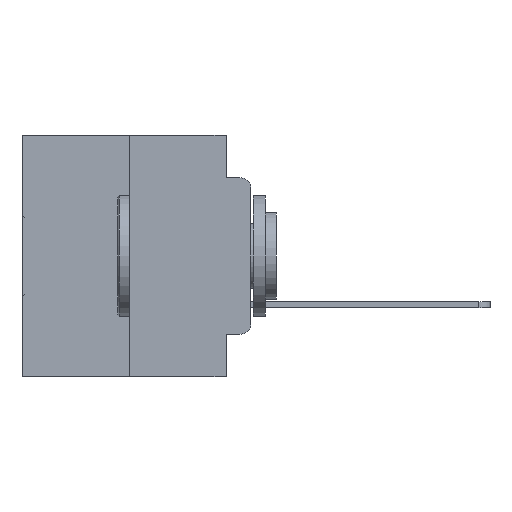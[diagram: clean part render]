
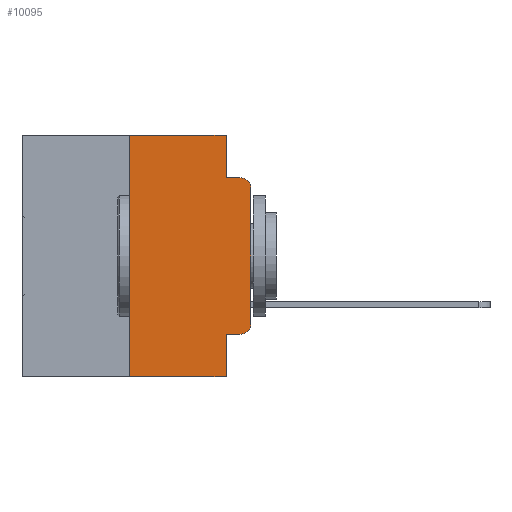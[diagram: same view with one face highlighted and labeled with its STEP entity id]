
A CAD part, left-side view. The second image highlights one B-rep face of the part: STEP entity #10095.
In plain terms, the highlighted planar face has unit normal (-1, 0, 0).
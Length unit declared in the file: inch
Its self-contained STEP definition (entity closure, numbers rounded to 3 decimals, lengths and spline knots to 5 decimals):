
#106 = DIRECTION ( 'NONE',  ( 0., 0., -1. ) ) ;
#397 = CARTESIAN_POINT ( 'NONE',  ( 0., 0., -0.3915 ) ) ;
#846 = CARTESIAN_POINT ( 'NONE',  ( 0., 0.25, 0. ) ) ;
#1183 = CARTESIAN_POINT ( 'NONE',  ( 0., 0.473, 0. ) ) ;
#2488 = CIRCLE ( 'NONE', #30219, 0.02 ) ;
#3315 = CARTESIAN_POINT ( 'NONE',  ( 0., 0.051, 0. ) ) ;
#3366 = LINE ( 'NONE', #1183, #28882 ) ;
#3495 = PLANE ( 'NONE',  #21438 ) ;
#3623 = DIRECTION ( 'NONE',  ( 0., 0., 1. ) ) ;
#3727 = LINE ( 'NONE', #16017, #16813 ) ;
#4218 = VECTOR ( 'NONE', #6435, 39.37008 ) ;
#4271 = VERTEX_POINT ( 'NONE', #10151 ) ;
#4418 = VERTEX_POINT ( 'NONE', #397 ) ;
#6343 = CARTESIAN_POINT ( 'NONE',  ( 0., 0.051, -0.0885 ) ) ;
#6427 = EDGE_CURVE ( 'NONE', #24190, #14633, #23889, .T. ) ;
#6435 = DIRECTION ( 'NONE',  ( 0., -1., 0. ) ) ;
#6467 = EDGE_CURVE ( 'NONE', #20273, #17217, #3366, .T. ) ;
#8149 = CARTESIAN_POINT ( 'NONE',  ( 0., 0.051, -0.5 ) ) ;
#8828 = DIRECTION ( 'NONE',  ( 0., 0., -1. ) ) ;
#9585 = DIRECTION ( 'NONE',  ( -1., 0., 0. ) ) ;
#10095 = ADVANCED_FACE ( 'NONE', ( #21127 ), #3495, .F. ) ;
#10151 = CARTESIAN_POINT ( 'NONE',  ( 0., 0., -0.1085 ) ) ;
#11311 = EDGE_LOOP ( 'NONE', ( #19283, #19315, #19781, #19879, #20159, #20254, #20561, #20663, #20999, #21186 ) ) ;
#11604 = VERTEX_POINT ( 'NONE', #26144 ) ;
#12731 = EDGE_CURVE ( 'NONE', #24190, #28984, #3727, .T. ) ;
#13324 = CARTESIAN_POINT ( 'NONE',  ( 0., 0.25, 0. ) ) ;
#14471 = EDGE_CURVE ( 'NONE', #11604, #20273, #20248, .T. ) ;
#14633 = VERTEX_POINT ( 'NONE', #24631 ) ;
#15648 = VECTOR ( 'NONE', #20537, 39.37008 ) ;
#15841 = DIRECTION ( 'NONE',  ( -1., 0., 0. ) ) ;
#16017 = CARTESIAN_POINT ( 'NONE',  ( 0., 0.051, 0. ) ) ;
#16194 = EDGE_CURVE ( 'NONE', #17217, #27124, #18966, .T. ) ;
#16813 = VECTOR ( 'NONE', #25944, 39.37008 ) ;
#17217 = VERTEX_POINT ( 'NONE', #3315 ) ;
#17726 = EDGE_CURVE ( 'NONE', #11604, #28984, #28880, .T. ) ;
#18016 = LINE ( 'NONE', #29142, #23846 ) ;
#18966 = LINE ( 'NONE', #23580, #24802 ) ;
#19283 = ORIENTED_EDGE ( 'NONE', *, *, #24597, .T. ) ;
#19315 = ORIENTED_EDGE ( 'NONE', *, *, #22913, .T. ) ;
#19781 = ORIENTED_EDGE ( 'NONE', *, *, #21266, .F. ) ;
#19879 = ORIENTED_EDGE ( 'NONE', *, *, #16194, .F. ) ;
#20159 = ORIENTED_EDGE ( 'NONE', *, *, #6467, .F. ) ;
#20248 = LINE ( 'NONE', #846, #26020 ) ;
#20254 = ORIENTED_EDGE ( 'NONE', *, *, #14471, .F. ) ;
#20273 = VERTEX_POINT ( 'NONE', #13324 ) ;
#20537 = DIRECTION ( 'NONE',  ( 0., -1., 0. ) ) ;
#20561 = ORIENTED_EDGE ( 'NONE', *, *, #17726, .T. ) ;
#20663 = ORIENTED_EDGE ( 'NONE', *, *, #12731, .F. ) ;
#20721 = VERTEX_POINT ( 'NONE', #29922 ) ;
#20999 = ORIENTED_EDGE ( 'NONE', *, *, #6427, .T. ) ;
#21127 = FACE_OUTER_BOUND ( 'NONE', #11311, .T. ) ;
#21186 = ORIENTED_EDGE ( 'NONE', *, *, #22491, .T. ) ;
#21266 = EDGE_CURVE ( 'NONE', #27124, #20721, #24764, .T. ) ;
#21438 = AXIS2_PLACEMENT_3D ( 'NONE', #21564, #24071, #8828 ) ;
#21564 = CARTESIAN_POINT ( 'NONE',  ( 0., 0.473, 0. ) ) ;
#21772 = CARTESIAN_POINT ( 'NONE',  ( 0., 0.051, -0.4115 ) ) ;
#22491 = EDGE_CURVE ( 'NONE', #14633, #4418, #25058, .T. ) ;
#22913 = EDGE_CURVE ( 'NONE', #4271, #20721, #2488, .T. ) ;
#23580 = CARTESIAN_POINT ( 'NONE',  ( 0., 0.051, 0. ) ) ;
#23846 = VECTOR ( 'NONE', #24205, 39.37008 ) ;
#23889 = LINE ( 'NONE', #21772, #4218 ) ;
#24071 = DIRECTION ( 'NONE',  ( 1., 0., 0. ) ) ;
#24190 = VERTEX_POINT ( 'NONE', #30341 ) ;
#24205 = DIRECTION ( 'NONE',  ( 0., 0., 1. ) ) ;
#24564 = CARTESIAN_POINT ( 'NONE',  ( 0., 0.051, -0.0885 ) ) ;
#24597 = EDGE_CURVE ( 'NONE', #4418, #4271, #18016, .T. ) ;
#24631 = CARTESIAN_POINT ( 'NONE',  ( 0., 0.02, -0.4115 ) ) ;
#24764 = LINE ( 'NONE', #6343, #30508 ) ;
#24802 = VECTOR ( 'NONE', #106, 39.37008 ) ;
#24810 = CARTESIAN_POINT ( 'NONE',  ( 0., 0.02, -0.1085 ) ) ;
#25058 = CIRCLE ( 'NONE', #29188, 0.02 ) ;
#25497 = CARTESIAN_POINT ( 'NONE',  ( 0., 0.473, -0.5 ) ) ;
#25944 = DIRECTION ( 'NONE',  ( 0., 0., -1. ) ) ;
#26020 = VECTOR ( 'NONE', #3623, 39.37008 ) ;
#26144 = CARTESIAN_POINT ( 'NONE',  ( 0., 0.25, -0.5 ) ) ;
#27124 = VERTEX_POINT ( 'NONE', #24564 ) ;
#27253 = DIRECTION ( 'NONE',  ( 0., 0., -1. ) ) ;
#28880 = LINE ( 'NONE', #25497, #15648 ) ;
#28882 = VECTOR ( 'NONE', #29329, 39.37008 ) ;
#28984 = VERTEX_POINT ( 'NONE', #8149 ) ;
#29139 = DIRECTION ( 'NONE',  ( 0., -1., 0. ) ) ;
#29142 = CARTESIAN_POINT ( 'NONE',  ( 0., 0., 0. ) ) ;
#29188 = AXIS2_PLACEMENT_3D ( 'NONE', #30719, #15841, #33206 ) ;
#29329 = DIRECTION ( 'NONE',  ( 0., -1., 0. ) ) ;
#29922 = CARTESIAN_POINT ( 'NONE',  ( 0., 0.02, -0.0885 ) ) ;
#30219 = AXIS2_PLACEMENT_3D ( 'NONE', #24810, #9585, #27253 ) ;
#30341 = CARTESIAN_POINT ( 'NONE',  ( 0., 0.051, -0.4115 ) ) ;
#30508 = VECTOR ( 'NONE', #29139, 39.37008 ) ;
#30719 = CARTESIAN_POINT ( 'NONE',  ( 0., 0.02, -0.3915 ) ) ;
#33206 = DIRECTION ( 'NONE',  ( 0., 0., -1. ) ) ;
